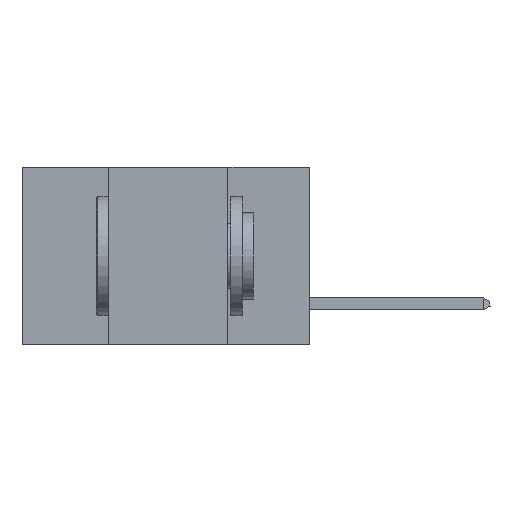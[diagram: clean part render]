
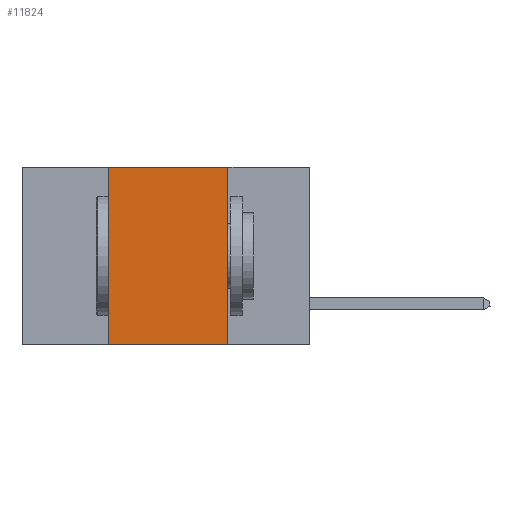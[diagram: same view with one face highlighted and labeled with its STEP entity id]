
A CAD part, left-side view. The second image highlights one B-rep face of the part: STEP entity #11824.
In plain terms, the highlighted planar face has unit normal (-1, 0, 0).
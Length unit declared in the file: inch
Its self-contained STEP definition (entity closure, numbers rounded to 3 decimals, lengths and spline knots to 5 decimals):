
#1995 = CARTESIAN_POINT ( 'NONE',  ( 0., 0.42, 0. ) ) ;
#2048 = EDGE_CURVE ( 'NONE', #10278, #13772, #17004, .T. ) ;
#2546 = DIRECTION ( 'NONE',  ( 0., 0., 1. ) ) ;
#3944 = CARTESIAN_POINT ( 'NONE',  ( 0., 0.17, 0. ) ) ;
#5008 = AXIS2_PLACEMENT_3D ( 'NONE', #23308, #12776, #5535 ) ;
#5535 = DIRECTION ( 'NONE',  ( 0., 0., -1. ) ) ;
#5949 = CARTESIAN_POINT ( 'NONE',  ( 0., 0.17, 0. ) ) ;
#6117 = DIRECTION ( 'NONE',  ( 0., 0., -1. ) ) ;
#6470 = ORIENTED_EDGE ( 'NONE', *, *, #13317, .T. ) ;
#6727 = LINE ( 'NONE', #11883, #21979 ) ;
#6996 = PLANE ( 'NONE',  #5008 ) ;
#7276 = CARTESIAN_POINT ( 'NONE',  ( 0., 0.17, -0.37 ) ) ;
#7540 = VECTOR ( 'NONE', #2546, 39.37008 ) ;
#8525 = CARTESIAN_POINT ( 'NONE',  ( 0., 0.42, -0.37 ) ) ;
#9317 = LINE ( 'NONE', #18904, #7540 ) ;
#9578 = EDGE_CURVE ( 'NONE', #13772, #22535, #21232, .T. ) ;
#10108 = VECTOR ( 'NONE', #11691, 39.37008 ) ;
#10278 = VERTEX_POINT ( 'NONE', #1995 ) ;
#11066 = VERTEX_POINT ( 'NONE', #8525 ) ;
#11476 = VECTOR ( 'NONE', #6117, 39.37008 ) ;
#11691 = DIRECTION ( 'NONE',  ( 0., -1., 0. ) ) ;
#11824 = ADVANCED_FACE ( 'NONE', ( #22571 ), #6996, .F. ) ;
#11883 = CARTESIAN_POINT ( 'NONE',  ( 0., 0.6, -0.37 ) ) ;
#12052 = ORIENTED_EDGE ( 'NONE', *, *, #2048, .F. ) ;
#12776 = DIRECTION ( 'NONE',  ( 1., 0., 0. ) ) ;
#13316 = EDGE_CURVE ( 'NONE', #11066, #10278, #9317, .T. ) ;
#13317 = EDGE_CURVE ( 'NONE', #11066, #22535, #6727, .T. ) ;
#13368 = CARTESIAN_POINT ( 'NONE',  ( 0., 0.6, 0. ) ) ;
#13772 = VERTEX_POINT ( 'NONE', #3944 ) ;
#14866 = ORIENTED_EDGE ( 'NONE', *, *, #9578, .F. ) ;
#17004 = LINE ( 'NONE', #13368, #10108 ) ;
#17426 = DIRECTION ( 'NONE',  ( 0., -1., 0. ) ) ;
#18904 = CARTESIAN_POINT ( 'NONE',  ( 0., 0.42, 0. ) ) ;
#19799 = ORIENTED_EDGE ( 'NONE', *, *, #13316, .F. ) ;
#21232 = LINE ( 'NONE', #5949, #11476 ) ;
#21979 = VECTOR ( 'NONE', #17426, 39.37008 ) ;
#22535 = VERTEX_POINT ( 'NONE', #7276 ) ;
#22571 = FACE_OUTER_BOUND ( 'NONE', #23227, .T. ) ;
#23227 = EDGE_LOOP ( 'NONE', ( #14866, #12052, #19799, #6470 ) ) ;
#23308 = CARTESIAN_POINT ( 'NONE',  ( 0., 0.6, 0. ) ) ;
